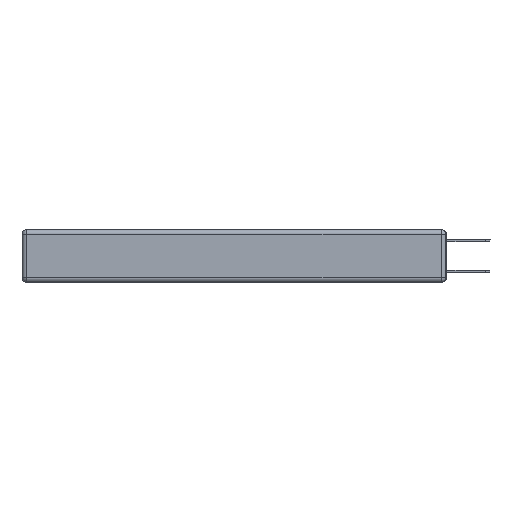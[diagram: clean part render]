
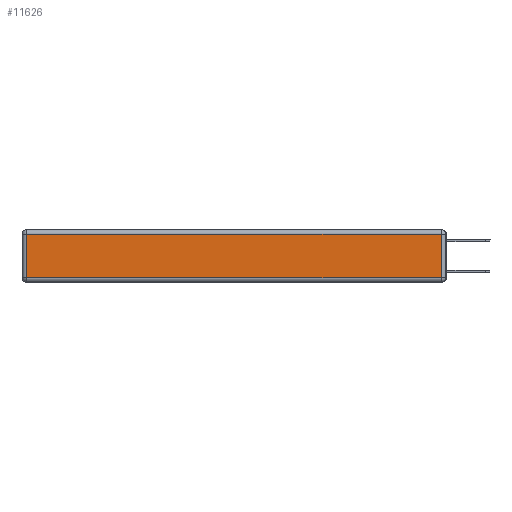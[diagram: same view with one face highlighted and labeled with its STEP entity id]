
A CAD part, left-side view. The second image highlights one B-rep face of the part: STEP entity #11626.
In plain terms, the highlighted planar face has unit normal (-1, 0, 0).
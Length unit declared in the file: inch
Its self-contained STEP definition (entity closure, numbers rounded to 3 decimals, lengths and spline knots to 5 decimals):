
#16 = CARTESIAN_POINT ( 'NONE',  ( 0., 0., -0.313 ) ) ;
#678 = VECTOR ( 'NONE', #11080, 39.37008 ) ;
#937 = CARTESIAN_POINT ( 'NONE',  ( 0., 0.03, -0.343 ) ) ;
#985 = ORIENTED_EDGE ( 'NONE', *, *, #12795, .T. ) ;
#1036 = DIRECTION ( 'NONE',  ( 0., 0., 1. ) ) ;
#1249 = DIRECTION ( 'NONE',  ( 0., -1., 0. ) ) ;
#2532 = VECTOR ( 'NONE', #10451, 39.37008 ) ;
#2772 = DIRECTION ( 'NONE',  ( 0., 0., -1. ) ) ;
#2939 = CARTESIAN_POINT ( 'NONE',  ( 0., 0., -0.343 ) ) ;
#3048 = VERTEX_POINT ( 'NONE', #6488 ) ;
#4014 = ORIENTED_EDGE ( 'NONE', *, *, #4491, .T. ) ;
#4138 = DIRECTION ( 'NONE',  ( -1., 0., 0. ) ) ;
#4230 = CARTESIAN_POINT ( 'NONE',  ( 0., 2.72, -0.313 ) ) ;
#4232 = ORIENTED_EDGE ( 'NONE', *, *, #12541, .T. ) ;
#4491 = EDGE_CURVE ( 'NONE', #3048, #10550, #13163, .T. ) ;
#6303 = LINE ( 'NONE', #937, #2532 ) ;
#6344 = CARTESIAN_POINT ( 'NONE',  ( 0., 0.03, -0.03 ) ) ;
#6374 = EDGE_LOOP ( 'NONE', ( #4232, #985, #9611, #4014 ) ) ;
#6488 = CARTESIAN_POINT ( 'NONE',  ( 0., 2.72, -0.03 ) ) ;
#7342 = LINE ( 'NONE', #11337, #678 ) ;
#7584 = VERTEX_POINT ( 'NONE', #9178 ) ;
#7867 = EDGE_CURVE ( 'NONE', #8587, #3048, #7342, .T. ) ;
#8221 = CARTESIAN_POINT ( 'NONE',  ( 0., 2.72, -0.343 ) ) ;
#8587 = VERTEX_POINT ( 'NONE', #6344 ) ;
#9178 = CARTESIAN_POINT ( 'NONE',  ( 0., 0.03, -0.313 ) ) ;
#9611 = ORIENTED_EDGE ( 'NONE', *, *, #7867, .T. ) ;
#10451 = DIRECTION ( 'NONE',  ( 0., 0., 1. ) ) ;
#10542 = VECTOR ( 'NONE', #2772, 39.37008 ) ;
#10550 = VERTEX_POINT ( 'NONE', #4230 ) ;
#11080 = DIRECTION ( 'NONE',  ( 0., 1., 0. ) ) ;
#11337 = CARTESIAN_POINT ( 'NONE',  ( 0., 2.75, -0.03 ) ) ;
#11524 = AXIS2_PLACEMENT_3D ( 'NONE', #2939, #4138, #1036 ) ;
#11626 = ADVANCED_FACE ( 'NONE', ( #12992 ), #14298, .T. ) ;
#12541 = EDGE_CURVE ( 'NONE', #10550, #7584, #16910, .T. ) ;
#12647 = VECTOR ( 'NONE', #1249, 39.37008 ) ;
#12795 = EDGE_CURVE ( 'NONE', #7584, #8587, #6303, .T. ) ;
#12992 = FACE_OUTER_BOUND ( 'NONE', #6374, .T. ) ;
#13163 = LINE ( 'NONE', #8221, #10542 ) ;
#14298 = PLANE ( 'NONE',  #11524 ) ;
#16910 = LINE ( 'NONE', #16, #12647 ) ;
